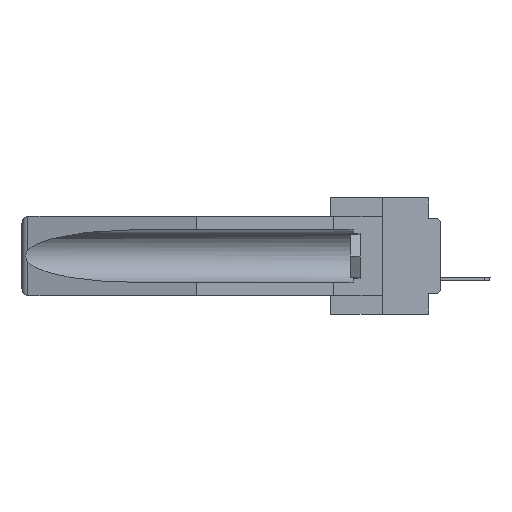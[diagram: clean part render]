
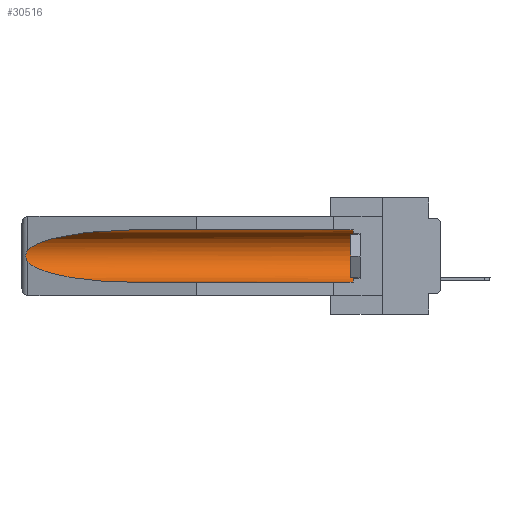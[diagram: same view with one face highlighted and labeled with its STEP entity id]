
A CAD part, left-side view. The second image highlights one B-rep face of the part: STEP entity #30516.
In plain terms, the highlighted cylindrical face has radius 2.857 mm (diameter 5.715 mm), a partial arc.
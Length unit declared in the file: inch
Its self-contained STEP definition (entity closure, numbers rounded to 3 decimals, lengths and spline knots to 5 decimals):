
#563 = CARTESIAN_POINT ( 'NONE',  ( 0.155, -0.30754, -0.284 ) ) ;
#2630 =( BOUNDED_CURVE ( )  B_SPLINE_CURVE ( 3, ( #24587, #35509, #25468, #11665 ),
 .UNSPECIFIED., .F., .F. ) 
 B_SPLINE_CURVE_WITH_KNOTS ( ( 4, 4 ),
 ( 0.1948, 1.5708 ),
 .UNSPECIFIED. ) 
 CURVE ( )  GEOMETRIC_REPRESENTATION_ITEM ( )  RATIONAL_B_SPLINE_CURVE ( ( 1., 0.848, 0.848, 1. ) ) 
 REPRESENTATION_ITEM ( '' )  );
#2683 = VECTOR ( 'NONE', #34680, 39.37008 ) ;
#3001 = CARTESIAN_POINT ( 'NONE',  ( 0.155, 1.07973, -0.284 ) ) ;
#3005 = ORIENTED_EDGE ( 'NONE', *, *, #18707, .T. ) ;
#3022 = CARTESIAN_POINT ( 'NONE',  ( 0.26597, 1.5296, -0.19026 ) ) ;
#3372 = CARTESIAN_POINT ( 'NONE',  ( 0.2675, 1.53308, -0.16763 ) ) ;
#3829 = AXIS2_PLACEMENT_3D ( 'NONE', #31928, #17483, #9028 ) ;
#4372 = CYLINDRICAL_SURFACE ( 'NONE', #26438, 0.1125 ) ;
#4529 = CARTESIAN_POINT ( 'NONE',  ( 0.26537, 1.52718, -0.14972 ) ) ;
#4868 = EDGE_CURVE ( 'NONE', #25693, #24691, #5514, .T. ) ;
#4941 =( BOUNDED_CURVE ( )  B_SPLINE_CURVE ( 3, ( #26605, #18032, #29119, #4529 ),
 .UNSPECIFIED., .F., .F. ) 
 B_SPLINE_CURVE_WITH_KNOTS ( ( 4, 4 ),
 ( 4.71239, 6.08839 ),
 .UNSPECIFIED. ) 
 CURVE ( )  GEOMETRIC_REPRESENTATION_ITEM ( )  RATIONAL_B_SPLINE_CURVE ( ( 1., 0.848, 0.848, 1. ) ) 
 REPRESENTATION_ITEM ( '' )  );
#5514 = B_SPLINE_CURVE_WITH_KNOTS ( 'NONE', 3,
 ( #16704, #30481, #5911, #30845, #3372, #28339, #11853, #22248, #3022, #25114 ),
 .UNSPECIFIED., .F., .F.,
 ( 4, 2, 2, 2, 4 ),
 ( 0., 0.00029, 0.00058, 0.00087, 0.00117 ),
 .UNSPECIFIED. ) ;
#5911 = CARTESIAN_POINT ( 'NONE',  ( 0.26654, 1.53092, -0.15636 ) ) ;
#7080 = CARTESIAN_POINT ( 'NONE',  ( 0.155, -0.30754, -0.1715 ) ) ;
#7582 = EDGE_CURVE ( 'NONE', #29631, #34990, #29597, .T. ) ;
#8617 = ORIENTED_EDGE ( 'NONE', *, *, #20643, .T. ) ;
#9028 = DIRECTION ( 'NONE',  ( 0., 0., 1. ) ) ;
#9920 = ORIENTED_EDGE ( 'NONE', *, *, #7582, .T. ) ;
#10476 = DIRECTION ( 'NONE',  ( 0., 1., 0. ) ) ;
#11554 = DIRECTION ( 'NONE',  ( 0., 1., 0. ) ) ;
#11665 = CARTESIAN_POINT ( 'NONE',  ( 0.155, 1.07973, -0.284 ) ) ;
#11742 = LINE ( 'NONE', #563, #11917 ) ;
#11853 = CARTESIAN_POINT ( 'NONE',  ( 0.2673, 1.53269, -0.17917 ) ) ;
#11917 = VECTOR ( 'NONE', #11554, 39.37008 ) ;
#12217 = CARTESIAN_POINT ( 'NONE',  ( 0.155, 0.126, -0.284 ) ) ;
#13066 = VERTEX_POINT ( 'NONE', #3001 ) ;
#15130 = ORIENTED_EDGE ( 'NONE', *, *, #16477, .T. ) ;
#15363 = FACE_OUTER_BOUND ( 'NONE', #21669, .T. ) ;
#16462 = CARTESIAN_POINT ( 'NONE',  ( 0.155, 1.07973, -0.059 ) ) ;
#16477 = EDGE_CURVE ( 'NONE', #34990, #32875, #34862, .T. ) ;
#16704 = CARTESIAN_POINT ( 'NONE',  ( 0.26537, 1.52718, -0.14972 ) ) ;
#17483 = DIRECTION ( 'NONE',  ( 0., -1., 0. ) ) ;
#17867 = DIRECTION ( 'NONE',  ( 0., 0., 1. ) ) ;
#18032 = CARTESIAN_POINT ( 'NONE',  ( 0.21114, 1.30732, -0.059 ) ) ;
#18490 = EDGE_CURVE ( 'NONE', #29631, #13066, #11742, .T. ) ;
#18707 = EDGE_CURVE ( 'NONE', #32875, #25693, #4941, .T. ) ;
#19071 = CARTESIAN_POINT ( 'NONE',  ( 0.155, -0.30754, -0.059 ) ) ;
#20643 = EDGE_CURVE ( 'NONE', #24691, #13066, #2630, .T. ) ;
#21669 = EDGE_LOOP ( 'NONE', ( #3005, #26478, #8617, #29039, #9920, #15130 ) ) ;
#22248 = CARTESIAN_POINT ( 'NONE',  ( 0.26655, 1.53094, -0.18657 ) ) ;
#23098 = CARTESIAN_POINT ( 'NONE',  ( 0.26537, 1.52718, -0.14972 ) ) ;
#24587 = CARTESIAN_POINT ( 'NONE',  ( 0.26537, 1.52718, -0.19328 ) ) ;
#24691 = VERTEX_POINT ( 'NONE', #26219 ) ;
#25114 = CARTESIAN_POINT ( 'NONE',  ( 0.26537, 1.52718, -0.19328 ) ) ;
#25468 = CARTESIAN_POINT ( 'NONE',  ( 0.21114, 1.30732, -0.284 ) ) ;
#25693 = VERTEX_POINT ( 'NONE', #23098 ) ;
#26219 = CARTESIAN_POINT ( 'NONE',  ( 0.26537, 1.52718, -0.19328 ) ) ;
#26438 = AXIS2_PLACEMENT_3D ( 'NONE', #7080, #10476, #17867 ) ;
#26478 = ORIENTED_EDGE ( 'NONE', *, *, #4868, .T. ) ;
#26605 = CARTESIAN_POINT ( 'NONE',  ( 0.155, 1.07973, -0.059 ) ) ;
#28339 = CARTESIAN_POINT ( 'NONE',  ( 0.2675, 1.53308, -0.17534 ) ) ;
#29039 = ORIENTED_EDGE ( 'NONE', *, *, #18490, .F. ) ;
#29119 = CARTESIAN_POINT ( 'NONE',  ( 0.25451, 1.48313, -0.09465 ) ) ;
#29398 = CARTESIAN_POINT ( 'NONE',  ( 0.155, 0.126, -0.059 ) ) ;
#29597 = CIRCLE ( 'NONE', #3829, 0.1125 ) ;
#29631 = VERTEX_POINT ( 'NONE', #12217 ) ;
#30481 = CARTESIAN_POINT ( 'NONE',  ( 0.26597, 1.52961, -0.15275 ) ) ;
#30516 = ADVANCED_FACE ( 'NONE', ( #15363 ), #4372, .F. ) ;
#30845 = CARTESIAN_POINT ( 'NONE',  ( 0.2673, 1.5327, -0.16383 ) ) ;
#31928 = CARTESIAN_POINT ( 'NONE',  ( 0.155, 0.126, -0.1715 ) ) ;
#32875 = VERTEX_POINT ( 'NONE', #16462 ) ;
#34680 = DIRECTION ( 'NONE',  ( 0., 1., 0. ) ) ;
#34862 = LINE ( 'NONE', #19071, #2683 ) ;
#34990 = VERTEX_POINT ( 'NONE', #29398 ) ;
#35509 = CARTESIAN_POINT ( 'NONE',  ( 0.25451, 1.48313, -0.24835 ) ) ;
